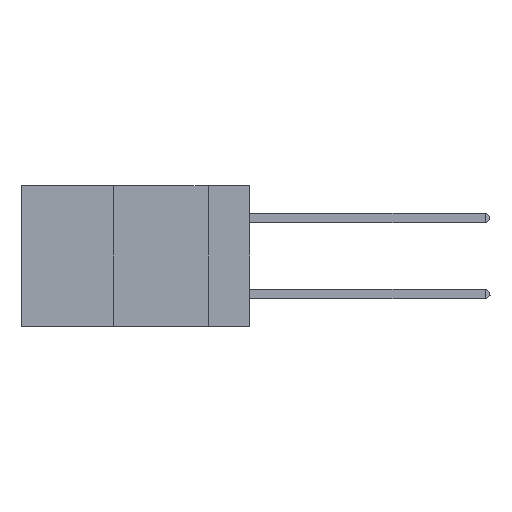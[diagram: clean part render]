
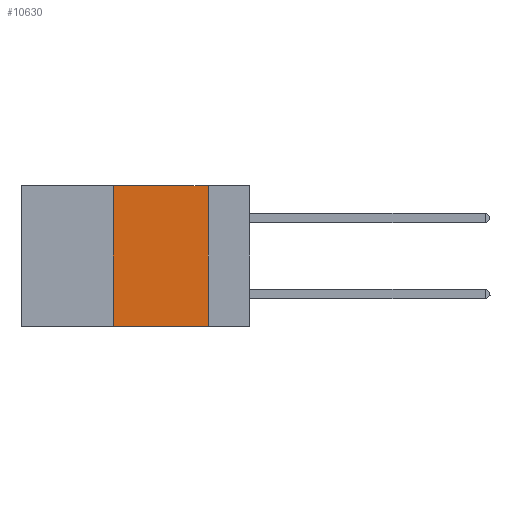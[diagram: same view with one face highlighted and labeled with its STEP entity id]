
A CAD part, left-side view. The second image highlights one B-rep face of the part: STEP entity #10630.
In plain terms, the highlighted planar face has unit normal (-1, 0, 0).
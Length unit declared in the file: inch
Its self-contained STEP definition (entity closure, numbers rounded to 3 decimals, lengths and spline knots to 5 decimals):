
#218 = CARTESIAN_POINT ( 'NONE',  ( 0., 0.36, 0. ) ) ;
#831 = CARTESIAN_POINT ( 'NONE',  ( 0., 0.6, 0. ) ) ;
#2514 = DIRECTION ( 'NONE',  ( 0., 0., -1. ) ) ;
#3040 = EDGE_CURVE ( 'NONE', #18142, #23110, #10724, .T. ) ;
#3160 = VERTEX_POINT ( 'NONE', #6893 ) ;
#3272 = VECTOR ( 'NONE', #6499, 39.37008 ) ;
#3612 = EDGE_CURVE ( 'NONE', #3160, #23110, #21644, .T. ) ;
#4679 = EDGE_LOOP ( 'NONE', ( #18551, #12749, #7779, #14312 ) ) ;
#5435 = DIRECTION ( 'NONE',  ( 0., 0., 1. ) ) ;
#6061 = LINE ( 'NONE', #831, #3272 ) ;
#6499 = DIRECTION ( 'NONE',  ( 0., -1., 0. ) ) ;
#6893 = CARTESIAN_POINT ( 'NONE',  ( 0., 0.36, -0.37 ) ) ;
#7590 = VECTOR ( 'NONE', #5435, 39.37008 ) ;
#7779 = ORIENTED_EDGE ( 'NONE', *, *, #9647, .F. ) ;
#8536 = DIRECTION ( 'NONE',  ( 1., 0., 0. ) ) ;
#8744 = VERTEX_POINT ( 'NONE', #17717 ) ;
#9647 = EDGE_CURVE ( 'NONE', #3160, #8744, #12064, .T. ) ;
#10008 = CARTESIAN_POINT ( 'NONE',  ( 0., 0.11, -0.37 ) ) ;
#10160 = VECTOR ( 'NONE', #2514, 39.37008 ) ;
#10630 = ADVANCED_FACE ( 'NONE', ( #11442 ), #17509, .F. ) ;
#10724 = LINE ( 'NONE', #11433, #10160 ) ;
#11433 = CARTESIAN_POINT ( 'NONE',  ( 0., 0.11, 0. ) ) ;
#11442 = FACE_OUTER_BOUND ( 'NONE', #4679, .T. ) ;
#12064 = LINE ( 'NONE', #218, #7590 ) ;
#12163 = CARTESIAN_POINT ( 'NONE',  ( 0., 0.11, 0. ) ) ;
#12749 = ORIENTED_EDGE ( 'NONE', *, *, #15370, .F. ) ;
#14312 = ORIENTED_EDGE ( 'NONE', *, *, #3612, .T. ) ;
#15370 = EDGE_CURVE ( 'NONE', #8744, #18142, #6061, .T. ) ;
#17434 = CARTESIAN_POINT ( 'NONE',  ( 0., 0.6, 0. ) ) ;
#17509 = PLANE ( 'NONE',  #21011 ) ;
#17717 = CARTESIAN_POINT ( 'NONE',  ( 0., 0.36, 0. ) ) ;
#18142 = VERTEX_POINT ( 'NONE', #12163 ) ;
#18365 = DIRECTION ( 'NONE',  ( 0., -1., 0. ) ) ;
#18551 = ORIENTED_EDGE ( 'NONE', *, *, #3040, .F. ) ;
#19400 = VECTOR ( 'NONE', #18365, 39.37008 ) ;
#21011 = AXIS2_PLACEMENT_3D ( 'NONE', #17434, #8536, #22858 ) ;
#21644 = LINE ( 'NONE', #21750, #19400 ) ;
#21750 = CARTESIAN_POINT ( 'NONE',  ( 0., 0.6, -0.37 ) ) ;
#22858 = DIRECTION ( 'NONE',  ( 0., 0., -1. ) ) ;
#23110 = VERTEX_POINT ( 'NONE', #10008 ) ;
